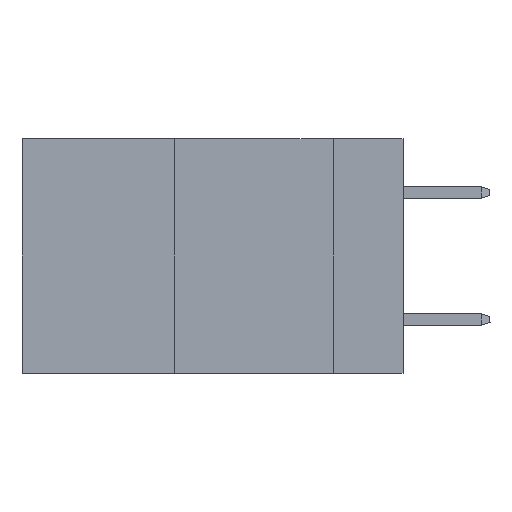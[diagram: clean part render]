
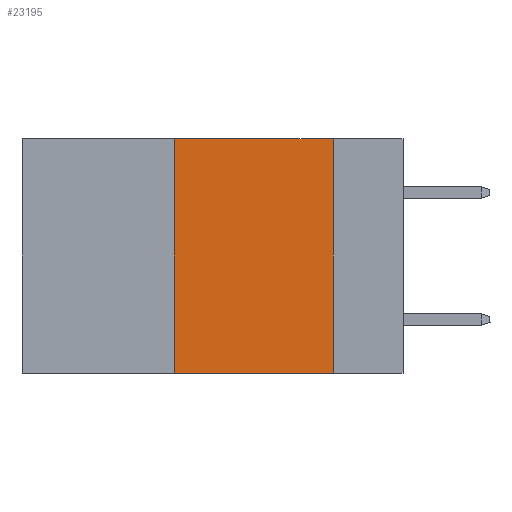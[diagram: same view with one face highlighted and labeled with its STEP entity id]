
A CAD part, left-side view. The second image highlights one B-rep face of the part: STEP entity #23195.
In plain terms, the highlighted planar face has unit normal (-1, 0, 0).
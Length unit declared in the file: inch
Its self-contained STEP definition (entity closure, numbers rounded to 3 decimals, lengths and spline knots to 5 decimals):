
#699 = CARTESIAN_POINT ( 'NONE',  ( 0., 0.6, -0.37 ) ) ;
#1518 = EDGE_CURVE ( 'NONE', #25170, #7074, #6872, .T. ) ;
#3328 = DIRECTION ( 'NONE',  ( 0., -1., 0. ) ) ;
#3459 = DIRECTION ( 'NONE',  ( 0., 0., 1. ) ) ;
#5078 = DIRECTION ( 'NONE',  ( 1., 0., 0. ) ) ;
#6225 = EDGE_CURVE ( 'NONE', #24751, #7074, #17702, .T. ) ;
#6377 = EDGE_CURVE ( 'NONE', #7646, #24751, #20962, .T. ) ;
#6872 = LINE ( 'NONE', #699, #27764 ) ;
#7074 = VERTEX_POINT ( 'NONE', #17499 ) ;
#7646 = VERTEX_POINT ( 'NONE', #10063 ) ;
#9348 = VECTOR ( 'NONE', #3459, 39.37008 ) ;
#9460 = VECTOR ( 'NONE', #3328, 39.37008 ) ;
#10063 = CARTESIAN_POINT ( 'NONE',  ( 0., 0.36, 0. ) ) ;
#11351 = CARTESIAN_POINT ( 'NONE',  ( 0., 0.11, 0. ) ) ;
#11388 = DIRECTION ( 'NONE',  ( 0., -1., 0. ) ) ;
#11798 = CARTESIAN_POINT ( 'NONE',  ( 0., 0.36, -0.37 ) ) ;
#11986 = EDGE_CURVE ( 'NONE', #25170, #7646, #20814, .T. ) ;
#13263 = FACE_OUTER_BOUND ( 'NONE', #15814, .T. ) ;
#13995 = VECTOR ( 'NONE', #22525, 39.37008 ) ;
#14183 = CARTESIAN_POINT ( 'NONE',  ( 0., 0.6, 0. ) ) ;
#14578 = ORIENTED_EDGE ( 'NONE', *, *, #1518, .T. ) ;
#15798 = PLANE ( 'NONE',  #24687 ) ;
#15814 = EDGE_LOOP ( 'NONE', ( #20247, #24453, #26523, #14578 ) ) ;
#16483 = CARTESIAN_POINT ( 'NONE',  ( 0., 0.11, 0. ) ) ;
#17499 = CARTESIAN_POINT ( 'NONE',  ( 0., 0.11, -0.37 ) ) ;
#17702 = LINE ( 'NONE', #11351, #13995 ) ;
#20247 = ORIENTED_EDGE ( 'NONE', *, *, #6225, .F. ) ;
#20814 = LINE ( 'NONE', #22788, #9348 ) ;
#20962 = LINE ( 'NONE', #14183, #9460 ) ;
#21893 = CARTESIAN_POINT ( 'NONE',  ( 0., 0.6, 0. ) ) ;
#22041 = DIRECTION ( 'NONE',  ( 0., 0., -1. ) ) ;
#22525 = DIRECTION ( 'NONE',  ( 0., 0., -1. ) ) ;
#22788 = CARTESIAN_POINT ( 'NONE',  ( 0., 0.36, 0. ) ) ;
#23195 = ADVANCED_FACE ( 'NONE', ( #13263 ), #15798, .F. ) ;
#24453 = ORIENTED_EDGE ( 'NONE', *, *, #6377, .F. ) ;
#24687 = AXIS2_PLACEMENT_3D ( 'NONE', #21893, #5078, #22041 ) ;
#24751 = VERTEX_POINT ( 'NONE', #16483 ) ;
#25170 = VERTEX_POINT ( 'NONE', #11798 ) ;
#26523 = ORIENTED_EDGE ( 'NONE', *, *, #11986, .F. ) ;
#27764 = VECTOR ( 'NONE', #11388, 39.37008 ) ;
